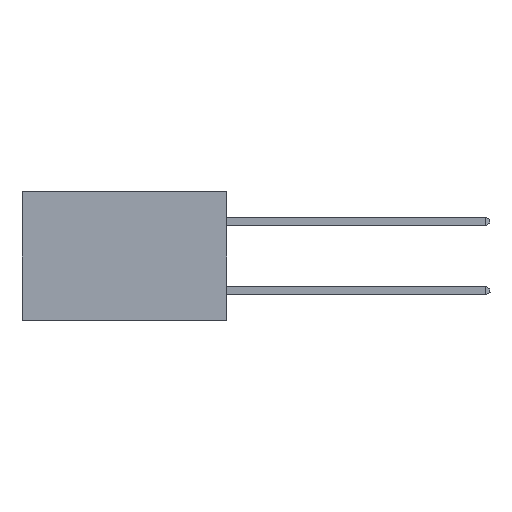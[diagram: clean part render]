
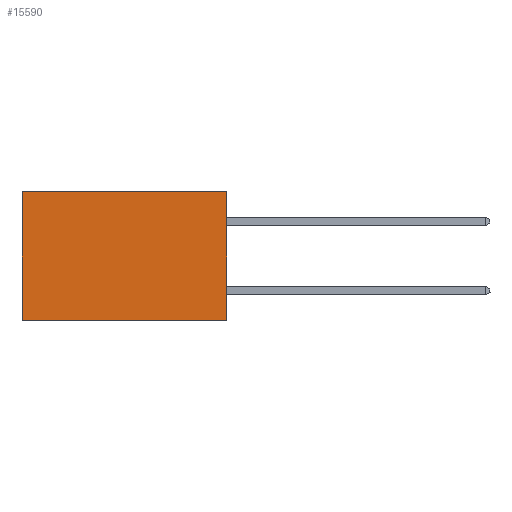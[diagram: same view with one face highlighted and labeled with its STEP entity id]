
A CAD part, left-side view. The second image highlights one B-rep face of the part: STEP entity #15590.
In plain terms, the highlighted planar face has unit normal (-1, 0, 0).
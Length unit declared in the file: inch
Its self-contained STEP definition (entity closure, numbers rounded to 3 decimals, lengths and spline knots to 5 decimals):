
#514 = CARTESIAN_POINT ( 'NONE',  ( 0.277, 0.59, 0. ) ) ;
#1955 = LINE ( 'NONE', #7580, #21454 ) ;
#2708 = VECTOR ( 'NONE', #8765, 39.37008 ) ;
#2826 = VECTOR ( 'NONE', #22470, 39.37008 ) ;
#2904 = EDGE_CURVE ( 'NONE', #14349, #6651, #12555, .T. ) ;
#3270 = LINE ( 'NONE', #8840, #2708 ) ;
#4225 = ORIENTED_EDGE ( 'NONE', *, *, #2904, .F. ) ;
#4346 = DIRECTION ( 'NONE',  ( 0., 0., -1. ) ) ;
#4875 = CARTESIAN_POINT ( 'NONE',  ( 0.277, 0., -0.37 ) ) ;
#5793 = CARTESIAN_POINT ( 'NONE',  ( 0.277, 0., -0.37 ) ) ;
#6565 = ORIENTED_EDGE ( 'NONE', *, *, #7910, .T. ) ;
#6651 = VERTEX_POINT ( 'NONE', #21450 ) ;
#7064 = DIRECTION ( 'NONE',  ( 1., 0., 0. ) ) ;
#7580 = CARTESIAN_POINT ( 'NONE',  ( 0.277, 0.59, -0.37 ) ) ;
#7910 = EDGE_CURVE ( 'NONE', #18793, #6651, #1955, .T. ) ;
#8765 = DIRECTION ( 'NONE',  ( 0., 1., 0. ) ) ;
#8840 = CARTESIAN_POINT ( 'NONE',  ( 0.277, 0., 0. ) ) ;
#10469 = EDGE_CURVE ( 'NONE', #18012, #18793, #3270, .T. ) ;
#11967 = LINE ( 'NONE', #4875, #21161 ) ;
#12504 = EDGE_LOOP ( 'NONE', ( #6565, #4225, #13973, #15625 ) ) ;
#12538 = PLANE ( 'NONE',  #12603 ) ;
#12555 = LINE ( 'NONE', #14106, #2826 ) ;
#12603 = AXIS2_PLACEMENT_3D ( 'NONE', #18092, #7064, #19948 ) ;
#13973 = ORIENTED_EDGE ( 'NONE', *, *, #16877, .F. ) ;
#14106 = CARTESIAN_POINT ( 'NONE',  ( 0.277, 0., -0.37 ) ) ;
#14349 = VERTEX_POINT ( 'NONE', #5793 ) ;
#15079 = FACE_OUTER_BOUND ( 'NONE', #12504, .T. ) ;
#15590 = ADVANCED_FACE ( 'NONE', ( #15079 ), #12538, .F. ) ;
#15625 = ORIENTED_EDGE ( 'NONE', *, *, #10469, .T. ) ;
#16877 = EDGE_CURVE ( 'NONE', #18012, #14349, #11967, .T. ) ;
#18012 = VERTEX_POINT ( 'NONE', #20566 ) ;
#18092 = CARTESIAN_POINT ( 'NONE',  ( 0.277, 0., -0.37 ) ) ;
#18793 = VERTEX_POINT ( 'NONE', #514 ) ;
#19574 = DIRECTION ( 'NONE',  ( 0., 0., -1. ) ) ;
#19948 = DIRECTION ( 'NONE',  ( 0., 0., -1. ) ) ;
#20566 = CARTESIAN_POINT ( 'NONE',  ( 0.277, 0., 0. ) ) ;
#21161 = VECTOR ( 'NONE', #19574, 39.37008 ) ;
#21450 = CARTESIAN_POINT ( 'NONE',  ( 0.277, 0.59, -0.37 ) ) ;
#21454 = VECTOR ( 'NONE', #4346, 39.37008 ) ;
#22470 = DIRECTION ( 'NONE',  ( 0., 1., 0. ) ) ;
